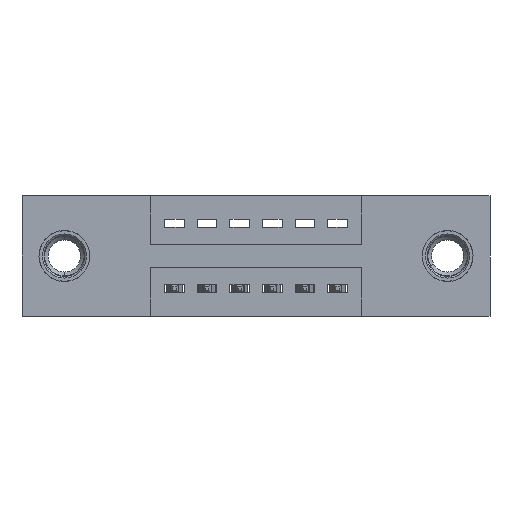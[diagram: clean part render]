
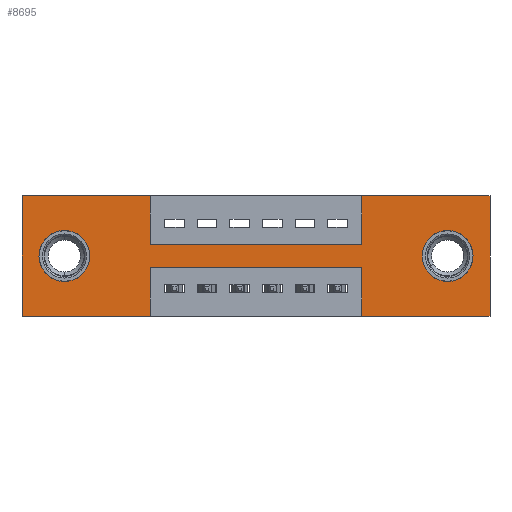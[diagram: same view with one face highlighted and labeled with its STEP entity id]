
A CAD part, front view. The second image highlights one B-rep face of the part: STEP entity #8695.
In plain terms, the highlighted planar face has unit normal (0, -1, 0).
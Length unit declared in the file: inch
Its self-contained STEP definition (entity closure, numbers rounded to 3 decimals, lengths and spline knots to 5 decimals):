
#14 = CARTESIAN_POINT ( 'NONE',  ( 0., 0., 0. ) ) ;
#155 = DIRECTION ( 'NONE',  ( 0., 0., 1. ) ) ;
#196 = LINE ( 'NONE', #7538, #322 ) ;
#264 = FACE_BOUND ( 'NONE', #8880, .T. ) ;
#291 = ORIENTED_EDGE ( 'NONE', *, *, #830, .F. ) ;
#315 = AXIS2_PLACEMENT_3D ( 'NONE', #1291, #10271, #2101 ) ;
#322 = VECTOR ( 'NONE', #155, 39.37008 ) ;
#323 = ORIENTED_EDGE ( 'NONE', *, *, #10218, .F. ) ;
#532 = CARTESIAN_POINT ( 'NONE',  ( 0.3925, 0., -0.22 ) ) ;
#602 = CARTESIAN_POINT ( 'NONE',  ( 1.305, 0., -0.185 ) ) ;
#615 = EDGE_CURVE ( 'NONE', #4569, #6657, #1654, .T. ) ;
#654 = DIRECTION ( 'NONE',  ( 0., 0., -1. ) ) ;
#739 = LINE ( 'NONE', #10519, #5718 ) ;
#792 = VERTEX_POINT ( 'NONE', #7523 ) ;
#830 = EDGE_CURVE ( 'NONE', #10347, #2269, #8030, .T. ) ;
#889 = EDGE_CURVE ( 'NONE', #792, #3715, #9317, .T. ) ;
#997 = DIRECTION ( 'NONE',  ( -1., 0., 0. ) ) ;
#1027 = DIRECTION ( 'NONE',  ( 0., 0., -1. ) ) ;
#1291 = CARTESIAN_POINT ( 'NONE',  ( 0.13, 0., -0.185 ) ) ;
#1387 = EDGE_LOOP ( 'NONE', ( #8839, #6610 ) ) ;
#1519 = CARTESIAN_POINT ( 'NONE',  ( 1.305, 0., -0.185 ) ) ;
#1520 = CARTESIAN_POINT ( 'NONE',  ( 0.3925, 0., -0.37 ) ) ;
#1525 = VECTOR ( 'NONE', #1027, 39.37008 ) ;
#1645 = ORIENTED_EDGE ( 'NONE', *, *, #2212, .F. ) ;
#1654 = CIRCLE ( 'NONE', #9401, 0.078 ) ;
#1794 = CARTESIAN_POINT ( 'NONE',  ( 1.305, 0., -0.263 ) ) ;
#1799 = VERTEX_POINT ( 'NONE', #7810 ) ;
#2101 = DIRECTION ( 'NONE',  ( 0., 0., 1. ) ) ;
#2131 = EDGE_CURVE ( 'NONE', #9658, #10347, #4320, .T. ) ;
#2212 = EDGE_CURVE ( 'NONE', #9151, #5757, #9149, .T. ) ;
#2269 = VERTEX_POINT ( 'NONE', #5508 ) ;
#2275 = EDGE_CURVE ( 'NONE', #5757, #8577, #4311, .T. ) ;
#2400 = DIRECTION ( 'NONE',  ( 0., 0., 1. ) ) ;
#2501 = VERTEX_POINT ( 'NONE', #14 ) ;
#2521 = PLANE ( 'NONE',  #2631 ) ;
#2631 = AXIS2_PLACEMENT_3D ( 'NONE', #9798, #5833, #4129 ) ;
#2773 = EDGE_CURVE ( 'NONE', #3767, #3719, #7607, .T. ) ;
#3039 = VECTOR ( 'NONE', #2400, 39.37008 ) ;
#3124 = CARTESIAN_POINT ( 'NONE',  ( 1.0425, 0., 0. ) ) ;
#3135 = DIRECTION ( 'NONE',  ( 0., 1., 0. ) ) ;
#3145 = DIRECTION ( 'NONE',  ( 0., 1., 0. ) ) ;
#3221 = CARTESIAN_POINT ( 'NONE',  ( 1.0425, 0., -0.22 ) ) ;
#3322 = CARTESIAN_POINT ( 'NONE',  ( 0.3925, 0., -0.37 ) ) ;
#3325 = CARTESIAN_POINT ( 'NONE',  ( 0., 0., -0.37 ) ) ;
#3495 = ORIENTED_EDGE ( 'NONE', *, *, #10245, .F. ) ;
#3715 = VERTEX_POINT ( 'NONE', #4574 ) ;
#3719 = VERTEX_POINT ( 'NONE', #8799 ) ;
#3734 = ORIENTED_EDGE ( 'NONE', *, *, #6820, .F. ) ;
#3767 = VERTEX_POINT ( 'NONE', #5495 ) ;
#4129 = DIRECTION ( 'NONE',  ( 0., 0., -1. ) ) ;
#4183 = CARTESIAN_POINT ( 'NONE',  ( 0.3925, 0., 0. ) ) ;
#4311 = LINE ( 'NONE', #3322, #6336 ) ;
#4320 = LINE ( 'NONE', #9357, #8394 ) ;
#4381 = CARTESIAN_POINT ( 'NONE',  ( 0.3925, 0., -0.15 ) ) ;
#4478 = ORIENTED_EDGE ( 'NONE', *, *, #9841, .T. ) ;
#4485 = DIRECTION ( 'NONE',  ( 0., 0., -1. ) ) ;
#4569 = VERTEX_POINT ( 'NONE', #6310 ) ;
#4574 = CARTESIAN_POINT ( 'NONE',  ( 0.3925, 0., -0.15 ) ) ;
#4686 = DIRECTION ( 'NONE',  ( 1., 0., 0. ) ) ;
#4771 = LINE ( 'NONE', #9568, #5648 ) ;
#4791 = AXIS2_PLACEMENT_3D ( 'NONE', #1519, #3135, #654 ) ;
#4887 = EDGE_CURVE ( 'NONE', #8577, #1799, #6842, .T. ) ;
#5069 = VECTOR ( 'NONE', #997, 39.37008 ) ;
#5310 = EDGE_CURVE ( 'NONE', #6657, #4569, #8376, .T. ) ;
#5495 = CARTESIAN_POINT ( 'NONE',  ( 0.13, 0., -0.263 ) ) ;
#5508 = CARTESIAN_POINT ( 'NONE',  ( 1.0425, 0., -0.37 ) ) ;
#5535 = EDGE_CURVE ( 'NONE', #1799, #2501, #196, .T. ) ;
#5648 = VECTOR ( 'NONE', #4686, 39.37008 ) ;
#5667 = ORIENTED_EDGE ( 'NONE', *, *, #7965, .F. ) ;
#5713 = CARTESIAN_POINT ( 'NONE',  ( 1.0425, 0., 0. ) ) ;
#5718 = VECTOR ( 'NONE', #9020, 39.37008 ) ;
#5757 = VERTEX_POINT ( 'NONE', #10170 ) ;
#5816 = CARTESIAN_POINT ( 'NONE',  ( 0., 0., -0.37 ) ) ;
#5833 = DIRECTION ( 'NONE',  ( 0., -1., 0. ) ) ;
#6171 = EDGE_CURVE ( 'NONE', #3715, #8362, #10137, .T. ) ;
#6308 = DIRECTION ( 'NONE',  ( 0., 1., 0. ) ) ;
#6310 = CARTESIAN_POINT ( 'NONE',  ( 1.305, 0., -0.107 ) ) ;
#6336 = VECTOR ( 'NONE', #8201, 39.37008 ) ;
#6511 = ORIENTED_EDGE ( 'NONE', *, *, #2773, .T. ) ;
#6610 = ORIENTED_EDGE ( 'NONE', *, *, #5310, .T. ) ;
#6657 = VERTEX_POINT ( 'NONE', #1794 ) ;
#6705 = CARTESIAN_POINT ( 'NONE',  ( 1.0425, 0., -0.37 ) ) ;
#6764 = FACE_BOUND ( 'NONE', #1387, .T. ) ;
#6820 = EDGE_CURVE ( 'NONE', #2269, #9151, #9230, .T. ) ;
#6842 = LINE ( 'NONE', #5816, #5069 ) ;
#6958 = ORIENTED_EDGE ( 'NONE', *, *, #889, .F. ) ;
#7071 = ORIENTED_EDGE ( 'NONE', *, *, #4887, .F. ) ;
#7089 = ORIENTED_EDGE ( 'NONE', *, *, #2275, .F. ) ;
#7123 = DIRECTION ( 'NONE',  ( 0., 0., -1. ) ) ;
#7186 = CARTESIAN_POINT ( 'NONE',  ( 0.13, 0., -0.185 ) ) ;
#7194 = EDGE_LOOP ( 'NONE', ( #7089, #1645, #3734, #291, #8001, #5667, #323, #8125, #6958, #3495, #9829, #7071 ) ) ;
#7241 = AXIS2_PLACEMENT_3D ( 'NONE', #7186, #3145, #10442 ) ;
#7273 = FACE_OUTER_BOUND ( 'NONE', #7194, .T. ) ;
#7523 = CARTESIAN_POINT ( 'NONE',  ( 0.3925, 0., 0. ) ) ;
#7538 = CARTESIAN_POINT ( 'NONE',  ( 0., 0., 0. ) ) ;
#7607 = CIRCLE ( 'NONE', #315, 0.078 ) ;
#7810 = CARTESIAN_POINT ( 'NONE',  ( 0., 0., -0.37 ) ) ;
#7835 = VECTOR ( 'NONE', #8833, 39.37008 ) ;
#7895 = CIRCLE ( 'NONE', #7241, 0.078 ) ;
#7965 = EDGE_CURVE ( 'NONE', #9227, #9658, #4771, .T. ) ;
#8001 = ORIENTED_EDGE ( 'NONE', *, *, #2131, .F. ) ;
#8030 = LINE ( 'NONE', #3325, #9954 ) ;
#8125 = ORIENTED_EDGE ( 'NONE', *, *, #6171, .F. ) ;
#8136 = LINE ( 'NONE', #5713, #3039 ) ;
#8201 = DIRECTION ( 'NONE',  ( 0., 0., -1. ) ) ;
#8305 = DIRECTION ( 'NONE',  ( -1., 0., 0. ) ) ;
#8362 = VERTEX_POINT ( 'NONE', #9119 ) ;
#8376 = CIRCLE ( 'NONE', #4791, 0.078 ) ;
#8394 = VECTOR ( 'NONE', #4485, 39.37008 ) ;
#8429 = DIRECTION ( 'NONE',  ( 1., 0., 0. ) ) ;
#8491 = CARTESIAN_POINT ( 'NONE',  ( 1.435, 0., -0.37 ) ) ;
#8521 = VECTOR ( 'NONE', #8609, 39.37008 ) ;
#8536 = CARTESIAN_POINT ( 'NONE',  ( 1.435, 0., 0. ) ) ;
#8577 = VERTEX_POINT ( 'NONE', #1520 ) ;
#8609 = DIRECTION ( 'NONE',  ( -1., 0., 0. ) ) ;
#8695 = ADVANCED_FACE ( 'NONE', ( #6764, #264, #7273 ), #2521, .T. ) ;
#8799 = CARTESIAN_POINT ( 'NONE',  ( 0.13, 0., -0.107 ) ) ;
#8833 = DIRECTION ( 'NONE',  ( 0., 0., 1. ) ) ;
#8839 = ORIENTED_EDGE ( 'NONE', *, *, #615, .T. ) ;
#8880 = EDGE_LOOP ( 'NONE', ( #4478, #6511 ) ) ;
#9020 = DIRECTION ( 'NONE',  ( 1., 0., 0. ) ) ;
#9119 = CARTESIAN_POINT ( 'NONE',  ( 1.0425, 0., -0.15 ) ) ;
#9149 = LINE ( 'NONE', #532, #8521 ) ;
#9151 = VERTEX_POINT ( 'NONE', #3221 ) ;
#9227 = VERTEX_POINT ( 'NONE', #3124 ) ;
#9230 = LINE ( 'NONE', #6705, #7835 ) ;
#9317 = LINE ( 'NONE', #4183, #1525 ) ;
#9357 = CARTESIAN_POINT ( 'NONE',  ( 1.435, 0., 0. ) ) ;
#9401 = AXIS2_PLACEMENT_3D ( 'NONE', #602, #6308, #7123 ) ;
#9568 = CARTESIAN_POINT ( 'NONE',  ( 0., 0., 0. ) ) ;
#9658 = VERTEX_POINT ( 'NONE', #8536 ) ;
#9798 = CARTESIAN_POINT ( 'NONE',  ( 0., 0., -0.37 ) ) ;
#9829 = ORIENTED_EDGE ( 'NONE', *, *, #5535, .F. ) ;
#9841 = EDGE_CURVE ( 'NONE', #3719, #3767, #7895, .T. ) ;
#9954 = VECTOR ( 'NONE', #8305, 39.37008 ) ;
#10137 = LINE ( 'NONE', #4381, #10390 ) ;
#10170 = CARTESIAN_POINT ( 'NONE',  ( 0.3925, 0., -0.22 ) ) ;
#10218 = EDGE_CURVE ( 'NONE', #8362, #9227, #8136, .T. ) ;
#10245 = EDGE_CURVE ( 'NONE', #2501, #792, #739, .T. ) ;
#10271 = DIRECTION ( 'NONE',  ( 0., 1., 0. ) ) ;
#10347 = VERTEX_POINT ( 'NONE', #8491 ) ;
#10390 = VECTOR ( 'NONE', #8429, 39.37008 ) ;
#10442 = DIRECTION ( 'NONE',  ( 0., 0., 1. ) ) ;
#10519 = CARTESIAN_POINT ( 'NONE',  ( 0., 0., 0. ) ) ;
